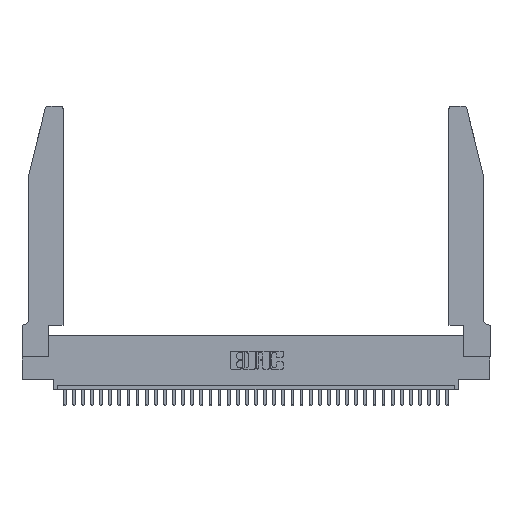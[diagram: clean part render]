
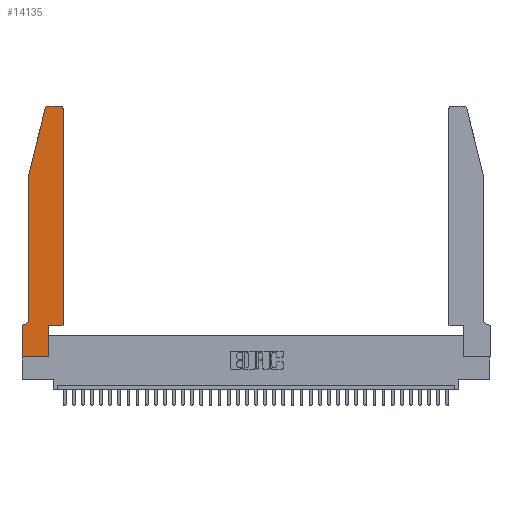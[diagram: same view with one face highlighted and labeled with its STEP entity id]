
A CAD part, top view. The second image highlights one B-rep face of the part: STEP entity #14135.
In plain terms, the highlighted planar face has unit normal (0, 0, 1).
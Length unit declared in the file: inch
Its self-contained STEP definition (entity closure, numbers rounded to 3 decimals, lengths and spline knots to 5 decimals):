
#110 = CARTESIAN_POINT ( 'NONE',  ( 0., 0., 0.37 ) ) ;
#759 = LINE ( 'NONE', #8798, #10707 ) ;
#855 = DIRECTION ( 'NONE',  ( 1., 0., 0. ) ) ;
#1043 = ORIENTED_EDGE ( 'NONE', *, *, #14158, .T. ) ;
#1550 = EDGE_CURVE ( 'NONE', #3301, #4084, #30309, .T. ) ;
#1642 = DIRECTION ( 'NONE',  ( -1., 0., 0. ) ) ;
#1886 = VECTOR ( 'NONE', #1642, 39.37008 ) ;
#2453 = CARTESIAN_POINT ( 'NONE',  ( 0.0755, 2., 0.37 ) ) ;
#2559 = DIRECTION ( 'NONE',  ( -1., 0., 0. ) ) ;
#2789 = LINE ( 'NONE', #18890, #1886 ) ;
#2812 = VECTOR ( 'NONE', #32390, 39.37008 ) ;
#3295 = ORIENTED_EDGE ( 'NONE', *, *, #6612, .T. ) ;
#3301 = VERTEX_POINT ( 'NONE', #32669 ) ;
#3315 = VECTOR ( 'NONE', #2559, 39.37008 ) ;
#3377 = CARTESIAN_POINT ( 'NONE',  ( 0.4205, 2.72, 0.37 ) ) ;
#3724 = CARTESIAN_POINT ( 'NONE',  ( 0.4205, 2.75, 0.37 ) ) ;
#4027 = ORIENTED_EDGE ( 'NONE', *, *, #31558, .T. ) ;
#4084 = VERTEX_POINT ( 'NONE', #24109 ) ;
#4736 = VECTOR ( 'NONE', #36320, 39.37008 ) ;
#5013 = LINE ( 'NONE', #28384, #13085 ) ;
#5206 = VECTOR ( 'NONE', #32876, 39.37008 ) ;
#5306 = EDGE_CURVE ( 'NONE', #30546, #19384, #6865, .T. ) ;
#6159 = CIRCLE ( 'NONE', #17794, 0.07 ) ;
#6425 = DIRECTION ( 'NONE',  ( 1., 0., 0. ) ) ;
#6612 = EDGE_CURVE ( 'NONE', #4084, #30963, #5013, .T. ) ;
#6865 = LINE ( 'NONE', #17864, #2812 ) ;
#6995 = VERTEX_POINT ( 'NONE', #2453 ) ;
#7429 = LINE ( 'NONE', #9502, #5206 ) ;
#7663 = CIRCLE ( 'NONE', #8531, 0.03 ) ;
#8123 = EDGE_CURVE ( 'NONE', #30963, #32104, #759, .T. ) ;
#8531 = AXIS2_PLACEMENT_3D ( 'NONE', #25924, #34661, #17287 ) ;
#8798 = CARTESIAN_POINT ( 'NONE',  ( 0., 0., 0.37 ) ) ;
#9502 = CARTESIAN_POINT ( 'NONE',  ( 0.0755, 2., 0.37 ) ) ;
#9988 = VERTEX_POINT ( 'NONE', #32667 ) ;
#10707 = VECTOR ( 'NONE', #20256, 39.37008 ) ;
#11273 = DIRECTION ( 'NONE',  ( 0., -1., 0. ) ) ;
#11901 = DIRECTION ( 'NONE',  ( 0., -1., 0. ) ) ;
#12197 = CARTESIAN_POINT ( 'NONE',  ( 0., 0.35, 0.37 ) ) ;
#12316 = CARTESIAN_POINT ( 'NONE',  ( 0.0755, 0.42, 0.37 ) ) ;
#12347 = LINE ( 'NONE', #22338, #4736 ) ;
#12868 = ORIENTED_EDGE ( 'NONE', *, *, #23433, .T. ) ;
#13085 = VECTOR ( 'NONE', #11273, 39.37008 ) ;
#13431 = CARTESIAN_POINT ( 'NONE',  ( 0.284, 2.75, 0.37 ) ) ;
#13717 = EDGE_CURVE ( 'NONE', #25043, #26866, #2789, .T. ) ;
#14135 = ADVANCED_FACE ( 'NONE', ( #35092 ), #26784, .T. ) ;
#14158 = EDGE_CURVE ( 'NONE', #9988, #30546, #23910, .T. ) ;
#14184 = EDGE_LOOP ( 'NONE', ( #22293, #4027, #31797, #21862, #12868, #34924, #3295, #18311, #16234, #1043, #26452, #25904 ) ) ;
#14444 = CARTESIAN_POINT ( 'NONE',  ( 0.0755, 2., 0.37 ) ) ;
#16234 = ORIENTED_EDGE ( 'NONE', *, *, #17927, .T. ) ;
#16558 = CARTESIAN_POINT ( 'NONE',  ( 0.0755, 0.35, 0.37 ) ) ;
#17097 = DIRECTION ( 'NONE',  ( 0., 0., -1. ) ) ;
#17287 = DIRECTION ( 'NONE',  ( 1., 0., 0. ) ) ;
#17735 = CARTESIAN_POINT ( 'NONE',  ( 0.4505, 2.72, 0.37 ) ) ;
#17758 = CARTESIAN_POINT ( 'NONE',  ( 0.4505, 0.35, 0.37 ) ) ;
#17794 = AXIS2_PLACEMENT_3D ( 'NONE', #37002, #17097, #34480 ) ;
#17864 = CARTESIAN_POINT ( 'NONE',  ( 0.4505, 0.35, 0.37 ) ) ;
#17927 = EDGE_CURVE ( 'NONE', #32104, #9988, #12347, .T. ) ;
#18218 = VERTEX_POINT ( 'NONE', #12316 ) ;
#18311 = ORIENTED_EDGE ( 'NONE', *, *, #8123, .T. ) ;
#18890 = CARTESIAN_POINT ( 'NONE',  ( 0.2605, 2.75, 0.37 ) ) ;
#19384 = VERTEX_POINT ( 'NONE', #17735 ) ;
#19652 = VECTOR ( 'NONE', #11901, 39.37008 ) ;
#20256 = DIRECTION ( 'NONE',  ( 1., 0., 0. ) ) ;
#20675 = VERTEX_POINT ( 'NONE', #20840 ) ;
#20840 = CARTESIAN_POINT ( 'NONE',  ( 0.25487, 2.72718, 0.37 ) ) ;
#21084 = AXIS2_PLACEMENT_3D ( 'NONE', #3377, #29883, #24646 ) ;
#21542 = AXIS2_PLACEMENT_3D ( 'NONE', #12197, #26399, #6425 ) ;
#21862 = ORIENTED_EDGE ( 'NONE', *, *, #28332, .T. ) ;
#22293 = ORIENTED_EDGE ( 'NONE', *, *, #13717, .T. ) ;
#22338 = CARTESIAN_POINT ( 'NONE',  ( 0.2865, 0.35, 0.37 ) ) ;
#23003 = CIRCLE ( 'NONE', #21084, 0.03 ) ;
#23433 = EDGE_CURVE ( 'NONE', #18218, #3301, #6159, .T. ) ;
#23910 = LINE ( 'NONE', #17758, #27060 ) ;
#24075 = CARTESIAN_POINT ( 'NONE',  ( 0.4505, 0.35, 0.37 ) ) ;
#24109 = CARTESIAN_POINT ( 'NONE',  ( 0., 0.35, 0.37 ) ) ;
#24646 = DIRECTION ( 'NONE',  ( 1., 0., 0. ) ) ;
#25043 = VERTEX_POINT ( 'NONE', #3724 ) ;
#25904 = ORIENTED_EDGE ( 'NONE', *, *, #31723, .T. ) ;
#25924 = CARTESIAN_POINT ( 'NONE',  ( 0.284, 2.72, 0.37 ) ) ;
#26399 = DIRECTION ( 'NONE',  ( 0., 0., 1. ) ) ;
#26452 = ORIENTED_EDGE ( 'NONE', *, *, #5306, .T. ) ;
#26784 = PLANE ( 'NONE',  #21542 ) ;
#26866 = VERTEX_POINT ( 'NONE', #13431 ) ;
#27060 = VECTOR ( 'NONE', #855, 39.37008 ) ;
#28332 = EDGE_CURVE ( 'NONE', #6995, #18218, #31704, .T. ) ;
#28384 = CARTESIAN_POINT ( 'NONE',  ( 0., 0., 0.37 ) ) ;
#29883 = DIRECTION ( 'NONE',  ( 0., 0., 1. ) ) ;
#30309 = LINE ( 'NONE', #16558, #3315 ) ;
#30546 = VERTEX_POINT ( 'NONE', #24075 ) ;
#30963 = VERTEX_POINT ( 'NONE', #110 ) ;
#31140 = CARTESIAN_POINT ( 'NONE',  ( 0.2865, 0., 0.37 ) ) ;
#31558 = EDGE_CURVE ( 'NONE', #26866, #20675, #7663, .T. ) ;
#31704 = LINE ( 'NONE', #14444, #19652 ) ;
#31723 = EDGE_CURVE ( 'NONE', #19384, #25043, #23003, .T. ) ;
#31797 = ORIENTED_EDGE ( 'NONE', *, *, #34632, .T. ) ;
#32104 = VERTEX_POINT ( 'NONE', #31140 ) ;
#32390 = DIRECTION ( 'NONE',  ( 0., 1., 0. ) ) ;
#32667 = CARTESIAN_POINT ( 'NONE',  ( 0.2865, 0.35, 0.37 ) ) ;
#32669 = CARTESIAN_POINT ( 'NONE',  ( 0.0055, 0.35, 0.37 ) ) ;
#32876 = DIRECTION ( 'NONE',  ( -0.239, -0.971, 0. ) ) ;
#34480 = DIRECTION ( 'NONE',  ( -1., 0., 0. ) ) ;
#34632 = EDGE_CURVE ( 'NONE', #20675, #6995, #7429, .T. ) ;
#34661 = DIRECTION ( 'NONE',  ( 0., 0., 1. ) ) ;
#34924 = ORIENTED_EDGE ( 'NONE', *, *, #1550, .T. ) ;
#35092 = FACE_OUTER_BOUND ( 'NONE', #14184, .T. ) ;
#36320 = DIRECTION ( 'NONE',  ( 0., 1., 0. ) ) ;
#37002 = CARTESIAN_POINT ( 'NONE',  ( 0.0055, 0.42, 0.37 ) ) ;
